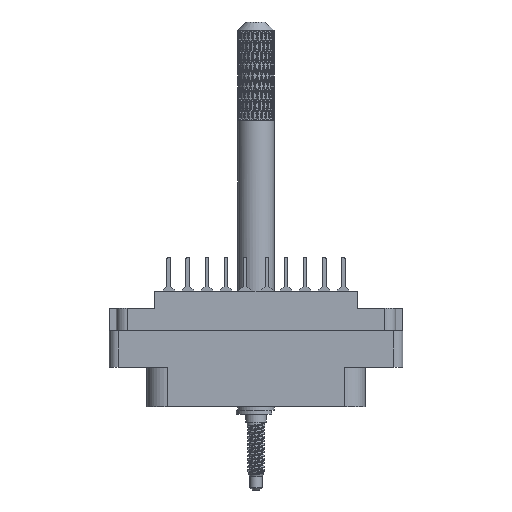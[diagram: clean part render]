
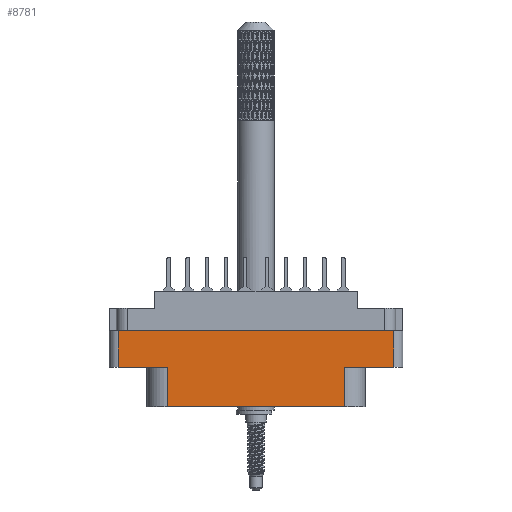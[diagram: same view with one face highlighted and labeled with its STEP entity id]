
A CAD part, front view. The second image highlights one B-rep face of the part: STEP entity #8781.
In plain terms, the highlighted planar face has unit normal (0, -1, 0).
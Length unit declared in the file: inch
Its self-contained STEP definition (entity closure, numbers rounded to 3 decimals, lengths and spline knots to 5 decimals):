
#555 = VECTOR ( 'NONE', #47060, 39.37008 ) ;
#1918 = EDGE_CURVE ( 'NONE', #62208, #98698, #42913, .T. ) ;
#1973 = VERTEX_POINT ( 'NONE', #34417 ) ;
#2489 = ORIENTED_EDGE ( 'NONE', *, *, #38501, .T. ) ;
#4946 = ORIENTED_EDGE ( 'NONE', *, *, #37842, .T. ) ;
#6717 = CARTESIAN_POINT ( 'NONE',  ( -0.938, -0.438, -0.789 ) ) ;
#8781 = ADVANCED_FACE ( 'NONE', ( #34694 ), #72164, .T. ) ;
#12213 = DIRECTION ( 'NONE',  ( 0., 0., 1. ) ) ;
#12572 = VECTOR ( 'NONE', #88072, 39.37008 ) ;
#13159 = CARTESIAN_POINT ( 'NONE',  ( -0.938, -0.438, -0.52 ) ) ;
#15436 = LINE ( 'NONE', #91128, #80326 ) ;
#17678 = LINE ( 'NONE', #83323, #82443 ) ;
#19051 = LINE ( 'NONE', #72072, #97757 ) ;
#21366 = CARTESIAN_POINT ( 'NONE',  ( 0.938, -0.438, -0.52 ) ) ;
#22014 = VECTOR ( 'NONE', #66446, 39.37008 ) ;
#23275 = VERTEX_POINT ( 'NONE', #89259 ) ;
#23655 = CARTESIAN_POINT ( 'NONE',  ( -1., -0.438, -0.789 ) ) ;
#29529 = ORIENTED_EDGE ( 'NONE', *, *, #52381, .T. ) ;
#30686 = CARTESIAN_POINT ( 'NONE',  ( -0.604, -0.438, -0.52 ) ) ;
#33053 = DIRECTION ( 'NONE',  ( 0., 0., -1. ) ) ;
#33295 = EDGE_CURVE ( 'NONE', #62208, #69617, #15436, .T. ) ;
#34417 = CARTESIAN_POINT ( 'NONE',  ( 0.604, -0.438, -0.52 ) ) ;
#34653 = VERTEX_POINT ( 'NONE', #30686 ) ;
#34694 = FACE_OUTER_BOUND ( 'NONE', #41411, .T. ) ;
#35285 = VERTEX_POINT ( 'NONE', #77568 ) ;
#37842 = EDGE_CURVE ( 'NONE', #23275, #1973, #17678, .T. ) ;
#38501 = EDGE_CURVE ( 'NONE', #35285, #23275, #38786, .T. ) ;
#38786 = LINE ( 'NONE', #95782, #12572 ) ;
#39168 = CARTESIAN_POINT ( 'NONE',  ( 0.938, -0.438, -0.268 ) ) ;
#40378 = DIRECTION ( 'NONE',  ( 0., 0., -1. ) ) ;
#41411 = EDGE_LOOP ( 'NONE', ( #89189, #49585, #88110, #29529, #2489, #4946, #98697, #73883 ) ) ;
#42913 = LINE ( 'NONE', #6717, #555 ) ;
#45973 = CARTESIAN_POINT ( 'NONE',  ( -0.938, -0.438, -0.268 ) ) ;
#47060 = DIRECTION ( 'NONE',  ( 0., 0., -1. ) ) ;
#48069 = EDGE_CURVE ( 'NONE', #98698, #34653, #83972, .T. ) ;
#49585 = ORIENTED_EDGE ( 'NONE', *, *, #1918, .T. ) ;
#52381 = EDGE_CURVE ( 'NONE', #34653, #35285, #71286, .T. ) ;
#56155 = CARTESIAN_POINT ( 'NONE',  ( 0., -0.438, -0.52 ) ) ;
#56255 = CARTESIAN_POINT ( 'NONE',  ( 0.938, -0.438, -0.789 ) ) ;
#56581 = VECTOR ( 'NONE', #75534, 39.37008 ) ;
#62208 = VERTEX_POINT ( 'NONE', #45973 ) ;
#63738 = VECTOR ( 'NONE', #33053, 39.37008 ) ;
#64047 = DIRECTION ( 'NONE',  ( -1., 0., 0. ) ) ;
#66446 = DIRECTION ( 'NONE',  ( 0., 0., 1. ) ) ;
#67092 = DIRECTION ( 'NONE',  ( 1., 0., 0. ) ) ;
#69617 = VERTEX_POINT ( 'NONE', #39168 ) ;
#70342 = EDGE_CURVE ( 'NONE', #84171, #1973, #19051, .T. ) ;
#71088 = LINE ( 'NONE', #56255, #22014 ) ;
#71286 = LINE ( 'NONE', #71833, #63738 ) ;
#71833 = CARTESIAN_POINT ( 'NONE',  ( -0.604, -0.438, -0.789 ) ) ;
#72072 = CARTESIAN_POINT ( 'NONE',  ( 0., -0.438, -0.52 ) ) ;
#72164 = PLANE ( 'NONE',  #92309 ) ;
#73883 = ORIENTED_EDGE ( 'NONE', *, *, #87791, .T. ) ;
#75534 = DIRECTION ( 'NONE',  ( 1., 0., 0. ) ) ;
#77568 = CARTESIAN_POINT ( 'NONE',  ( -0.604, -0.438, -0.789 ) ) ;
#79152 = DIRECTION ( 'NONE',  ( 0., -1., 0. ) ) ;
#80326 = VECTOR ( 'NONE', #67092, 39.37008 ) ;
#82443 = VECTOR ( 'NONE', #12213, 39.37008 ) ;
#83323 = CARTESIAN_POINT ( 'NONE',  ( 0.604, -0.438, -0.52 ) ) ;
#83972 = LINE ( 'NONE', #56155, #56581 ) ;
#84171 = VERTEX_POINT ( 'NONE', #21366 ) ;
#87791 = EDGE_CURVE ( 'NONE', #84171, #69617, #71088, .T. ) ;
#88072 = DIRECTION ( 'NONE',  ( 1., 0., 0. ) ) ;
#88110 = ORIENTED_EDGE ( 'NONE', *, *, #48069, .T. ) ;
#89189 = ORIENTED_EDGE ( 'NONE', *, *, #33295, .F. ) ;
#89259 = CARTESIAN_POINT ( 'NONE',  ( 0.604, -0.438, -0.789 ) ) ;
#91128 = CARTESIAN_POINT ( 'NONE',  ( 0., -0.438, -0.268 ) ) ;
#92309 = AXIS2_PLACEMENT_3D ( 'NONE', #23655, #79152, #40378 ) ;
#95782 = CARTESIAN_POINT ( 'NONE',  ( -1., -0.438, -0.789 ) ) ;
#97757 = VECTOR ( 'NONE', #64047, 39.37008 ) ;
#98697 = ORIENTED_EDGE ( 'NONE', *, *, #70342, .F. ) ;
#98698 = VERTEX_POINT ( 'NONE', #13159 ) ;
